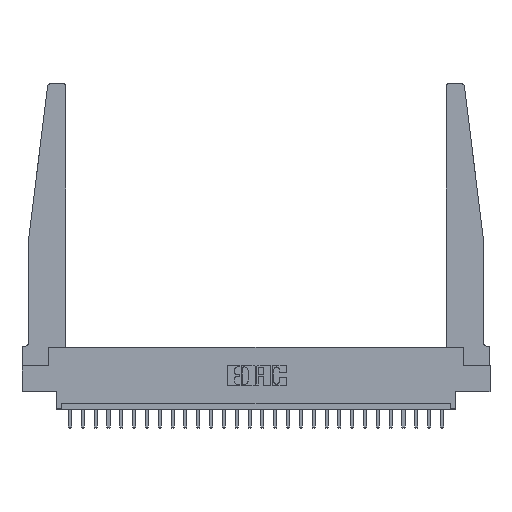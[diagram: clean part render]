
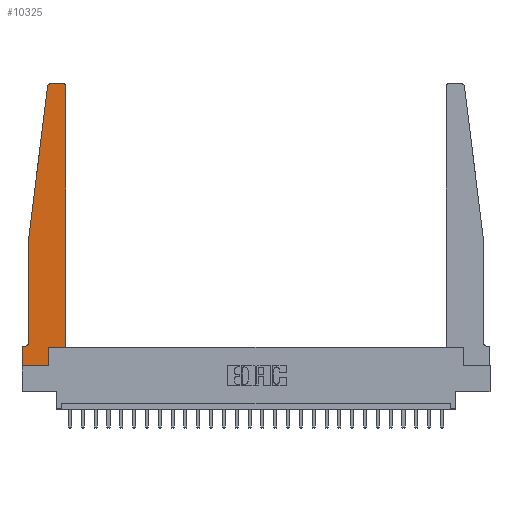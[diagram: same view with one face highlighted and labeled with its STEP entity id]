
A CAD part, top view. The second image highlights one B-rep face of the part: STEP entity #10325.
In plain terms, the highlighted planar face has unit normal (0, 0, 1).
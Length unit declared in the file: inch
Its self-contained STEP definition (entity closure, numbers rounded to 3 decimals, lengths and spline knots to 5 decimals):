
#24 = VERTEX_POINT ( 'NONE', #18183 ) ;
#62 = EDGE_CURVE ( 'NONE', #20244, #4072, #6630, .T. ) ;
#377 = DIRECTION ( 'NONE',  ( 0., -1., 0. ) ) ;
#611 = EDGE_CURVE ( 'NONE', #8414, #6124, #9998, .T. ) ;
#702 = VERTEX_POINT ( 'NONE', #14923 ) ;
#732 = ORIENTED_EDGE ( 'NONE', *, *, #25013, .T. ) ;
#954 = CARTESIAN_POINT ( 'NONE',  ( 0., 0., 0.37 ) ) ;
#1097 = ORIENTED_EDGE ( 'NONE', *, *, #13003, .T. ) ;
#1147 = EDGE_CURVE ( 'NONE', #20035, #10102, #21497, .T. ) ;
#1306 = CARTESIAN_POINT ( 'NONE',  ( 0.25, 2.75, 0.37 ) ) ;
#1310 = VECTOR ( 'NONE', #22607, 39.37008 ) ;
#1329 = DIRECTION ( 'NONE',  ( 0., 1., 0. ) ) ;
#1407 = DIRECTION ( 'NONE',  ( 1., 0., 0. ) ) ;
#1454 = CIRCLE ( 'NONE', #3385, 0.03 ) ;
#1684 = DIRECTION ( 'NONE',  ( 0., 0., 1. ) ) ;
#1688 = EDGE_CURVE ( 'NONE', #17100, #20244, #11443, .T. ) ;
#2336 = DIRECTION ( 'NONE',  ( 0., 0., 1. ) ) ;
#2480 = VERTEX_POINT ( 'NONE', #14019 ) ;
#2590 = VECTOR ( 'NONE', #12863, 39.37008 ) ;
#2739 = EDGE_CURVE ( 'NONE', #2480, #702, #7721, .T. ) ;
#3385 = AXIS2_PLACEMENT_3D ( 'NONE', #25182, #1684, #7853 ) ;
#3649 = CARTESIAN_POINT ( 'NONE',  ( 0.2605, 0., 0.37 ) ) ;
#3787 = CARTESIAN_POINT ( 'NONE',  ( 0.24675, 2.72367, 0.37 ) ) ;
#4072 = VERTEX_POINT ( 'NONE', #25008 ) ;
#4570 = ORIENTED_EDGE ( 'NONE', *, *, #2739, .T. ) ;
#5004 = CARTESIAN_POINT ( 'NONE',  ( 0.2605, 0.18, 0.37 ) ) ;
#5009 = VERTEX_POINT ( 'NONE', #3649 ) ;
#5035 = LINE ( 'NONE', #5004, #16311 ) ;
#5264 = CARTESIAN_POINT ( 'NONE',  ( 0., 0.1875, 0.37 ) ) ;
#5346 = PLANE ( 'NONE',  #21786 ) ;
#5719 = EDGE_CURVE ( 'NONE', #5009, #17100, #5035, .T. ) ;
#5857 = LINE ( 'NONE', #954, #10486 ) ;
#5899 = DIRECTION ( 'NONE',  ( -1., 0., 0. ) ) ;
#6093 = CARTESIAN_POINT ( 'NONE',  ( 0.27653, 2.75, 0.37 ) ) ;
#6124 = VERTEX_POINT ( 'NONE', #10537 ) ;
#6428 = ORIENTED_EDGE ( 'NONE', *, *, #8082, .T. ) ;
#6445 = EDGE_CURVE ( 'NONE', #702, #5009, #5857, .T. ) ;
#6630 = LINE ( 'NONE', #16632, #13057 ) ;
#7223 = ORIENTED_EDGE ( 'NONE', *, *, #62, .T. ) ;
#7721 = LINE ( 'NONE', #17819, #23243 ) ;
#7853 = DIRECTION ( 'NONE',  ( 1., 0., 0. ) ) ;
#7950 = LINE ( 'NONE', #13919, #19213 ) ;
#8082 = EDGE_CURVE ( 'NONE', #10102, #2480, #7950, .T. ) ;
#8105 = ORIENTED_EDGE ( 'NONE', *, *, #5719, .T. ) ;
#8319 = DIRECTION ( 'NONE',  ( 1., 0., 0. ) ) ;
#8414 = VERTEX_POINT ( 'NONE', #3787 ) ;
#8799 = ORIENTED_EDGE ( 'NONE', *, *, #22267, .T. ) ;
#8935 = AXIS2_PLACEMENT_3D ( 'NONE', #11982, #2336, #8319 ) ;
#9429 = DIRECTION ( 'NONE',  ( 1., 0., 0. ) ) ;
#9478 = CARTESIAN_POINT ( 'NONE',  ( 0.425, 0.18, 0.37 ) ) ;
#9998 = LINE ( 'NONE', #24404, #12099 ) ;
#10102 = VERTEX_POINT ( 'NONE', #10363 ) ;
#10325 = ADVANCED_FACE ( 'NONE', ( #22430 ), #5346, .T. ) ;
#10363 = CARTESIAN_POINT ( 'NONE',  ( 0.015, 0.1875, 0.37 ) ) ;
#10431 = CARTESIAN_POINT ( 'NONE',  ( 0.065, 0.2375, 0.37 ) ) ;
#10486 = VECTOR ( 'NONE', #9429, 39.37008 ) ;
#10537 = CARTESIAN_POINT ( 'NONE',  ( 0.065, 1.25, 0.37 ) ) ;
#11166 = DIRECTION ( 'NONE',  ( 0., 0., 1. ) ) ;
#11443 = LINE ( 'NONE', #22196, #2590 ) ;
#11677 = VECTOR ( 'NONE', #23608, 39.37008 ) ;
#11861 = CARTESIAN_POINT ( 'NONE',  ( 0.2605, 0.18, 0.37 ) ) ;
#11982 = CARTESIAN_POINT ( 'NONE',  ( 0.27653, 2.72, 0.37 ) ) ;
#12099 = VECTOR ( 'NONE', #24315, 39.37008 ) ;
#12240 = AXIS2_PLACEMENT_3D ( 'NONE', #19814, #23786, #5899 ) ;
#12794 = EDGE_CURVE ( 'NONE', #24, #16354, #19022, .T. ) ;
#12863 = DIRECTION ( 'NONE',  ( 1., 0., 0. ) ) ;
#13003 = EDGE_CURVE ( 'NONE', #6124, #20035, #16560, .T. ) ;
#13057 = VECTOR ( 'NONE', #1329, 39.37008 ) ;
#13919 = CARTESIAN_POINT ( 'NONE',  ( 0.065, 0.1875, 0.37 ) ) ;
#14019 = CARTESIAN_POINT ( 'NONE',  ( 0., 0.1875, 0.37 ) ) ;
#14291 = EDGE_LOOP ( 'NONE', ( #22771, #8799, #14686, #1097, #17618, #6428, #4570, #23433, #8105, #14693, #7223, #732 ) ) ;
#14686 = ORIENTED_EDGE ( 'NONE', *, *, #611, .T. ) ;
#14693 = ORIENTED_EDGE ( 'NONE', *, *, #1688, .T. ) ;
#14923 = CARTESIAN_POINT ( 'NONE',  ( 0., 0., 0.37 ) ) ;
#15900 = DIRECTION ( 'NONE',  ( -1., 0., 0. ) ) ;
#16311 = VECTOR ( 'NONE', #18630, 39.37008 ) ;
#16354 = VERTEX_POINT ( 'NONE', #6093 ) ;
#16560 = LINE ( 'NONE', #21653, #11677 ) ;
#16632 = CARTESIAN_POINT ( 'NONE',  ( 0.425, 0.18, 0.37 ) ) ;
#17100 = VERTEX_POINT ( 'NONE', #11861 ) ;
#17618 = ORIENTED_EDGE ( 'NONE', *, *, #1147, .T. ) ;
#17819 = CARTESIAN_POINT ( 'NONE',  ( 0., 0., 0.37 ) ) ;
#18183 = CARTESIAN_POINT ( 'NONE',  ( 0.395, 2.75, 0.37 ) ) ;
#18630 = DIRECTION ( 'NONE',  ( 0., 1., 0. ) ) ;
#19022 = LINE ( 'NONE', #1306, #1310 ) ;
#19213 = VECTOR ( 'NONE', #15900, 39.37008 ) ;
#19814 = CARTESIAN_POINT ( 'NONE',  ( 0.015, 0.2375, 0.37 ) ) ;
#20035 = VERTEX_POINT ( 'NONE', #10431 ) ;
#20244 = VERTEX_POINT ( 'NONE', #9478 ) ;
#21497 = CIRCLE ( 'NONE', #12240, 0.05 ) ;
#21653 = CARTESIAN_POINT ( 'NONE',  ( 0.065, 1.25, 0.37 ) ) ;
#21786 = AXIS2_PLACEMENT_3D ( 'NONE', #5264, #11166, #1407 ) ;
#22196 = CARTESIAN_POINT ( 'NONE',  ( 0.425, 0.18, 0.37 ) ) ;
#22267 = EDGE_CURVE ( 'NONE', #16354, #8414, #24128, .T. ) ;
#22430 = FACE_OUTER_BOUND ( 'NONE', #14291, .T. ) ;
#22607 = DIRECTION ( 'NONE',  ( -1., 0., 0. ) ) ;
#22771 = ORIENTED_EDGE ( 'NONE', *, *, #12794, .T. ) ;
#23243 = VECTOR ( 'NONE', #377, 39.37008 ) ;
#23433 = ORIENTED_EDGE ( 'NONE', *, *, #6445, .T. ) ;
#23608 = DIRECTION ( 'NONE',  ( 0., -1., 0. ) ) ;
#23786 = DIRECTION ( 'NONE',  ( 0., 0., -1. ) ) ;
#24128 = CIRCLE ( 'NONE', #8935, 0.03 ) ;
#24315 = DIRECTION ( 'NONE',  ( -0.122, -0.992, 0. ) ) ;
#24404 = CARTESIAN_POINT ( 'NONE',  ( 0.065, 1.25, 0.37 ) ) ;
#25008 = CARTESIAN_POINT ( 'NONE',  ( 0.425, 2.72, 0.37 ) ) ;
#25013 = EDGE_CURVE ( 'NONE', #4072, #24, #1454, .T. ) ;
#25182 = CARTESIAN_POINT ( 'NONE',  ( 0.395, 2.72, 0.37 ) ) ;
